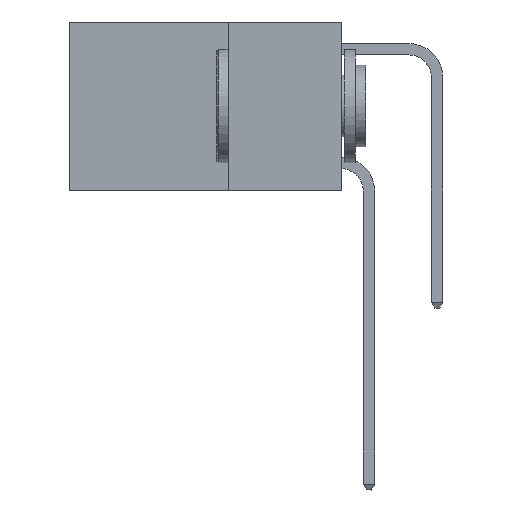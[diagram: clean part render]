
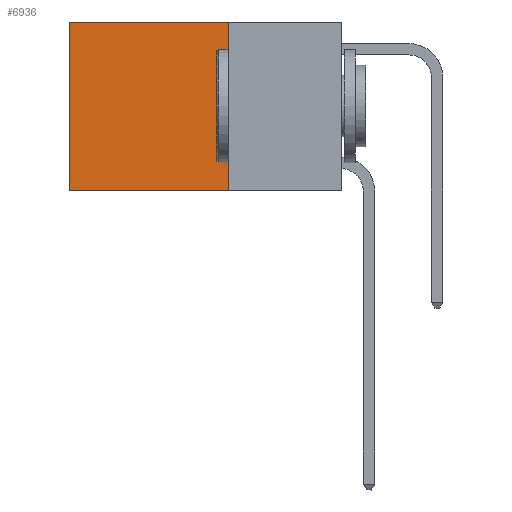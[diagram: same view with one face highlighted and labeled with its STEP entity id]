
A CAD part, left-side view. The second image highlights one B-rep face of the part: STEP entity #6936.
In plain terms, the highlighted planar face has unit normal (-1, 0, 0).
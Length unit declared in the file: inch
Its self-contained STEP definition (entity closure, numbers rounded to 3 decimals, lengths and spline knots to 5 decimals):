
#283 = CARTESIAN_POINT ( 'NONE',  ( 0.2625, 0.6, 0. ) ) ;
#607 = CARTESIAN_POINT ( 'NONE',  ( 0.2625, 0.25, 0. ) ) ;
#951 = CARTESIAN_POINT ( 'NONE',  ( 0.2625, 0.6, -0.37 ) ) ;
#1100 = VERTEX_POINT ( 'NONE', #7781 ) ;
#1145 = VERTEX_POINT ( 'NONE', #7537 ) ;
#1238 = DIRECTION ( 'NONE',  ( 1., 0., 0. ) ) ;
#1539 = VECTOR ( 'NONE', #5358, 39.37008 ) ;
#1725 = LINE ( 'NONE', #283, #9116 ) ;
#2464 = EDGE_CURVE ( 'NONE', #10876, #1145, #8487, .T. ) ;
#2500 = VERTEX_POINT ( 'NONE', #951 ) ;
#3255 = CARTESIAN_POINT ( 'NONE',  ( 0.2625, 0.25, 0. ) ) ;
#4139 = ORIENTED_EDGE ( 'NONE', *, *, #5189, .T. ) ;
#4160 = DIRECTION ( 'NONE',  ( 0., 1., 0. ) ) ;
#4683 = ORIENTED_EDGE ( 'NONE', *, *, #7695, .F. ) ;
#5189 = EDGE_CURVE ( 'NONE', #1100, #2500, #1725, .T. ) ;
#5267 = ORIENTED_EDGE ( 'NONE', *, *, #2464, .F. ) ;
#5355 = AXIS2_PLACEMENT_3D ( 'NONE', #10351, #1238, #7827 ) ;
#5358 = DIRECTION ( 'NONE',  ( 0., 1., 0. ) ) ;
#5372 = VECTOR ( 'NONE', #4160, 39.37008 ) ;
#5715 = ORIENTED_EDGE ( 'NONE', *, *, #9341, .T. ) ;
#5898 = DIRECTION ( 'NONE',  ( 0., 0., -1. ) ) ;
#6398 = VECTOR ( 'NONE', #10299, 39.37008 ) ;
#6750 = FACE_OUTER_BOUND ( 'NONE', #6798, .T. ) ;
#6798 = EDGE_LOOP ( 'NONE', ( #4139, #4683, #5267, #5715 ) ) ;
#6936 = ADVANCED_FACE ( 'NONE', ( #6750 ), #8650, .F. ) ;
#7046 = LINE ( 'NONE', #3255, #5372 ) ;
#7537 = CARTESIAN_POINT ( 'NONE',  ( 0.2625, 0.25, -0.37 ) ) ;
#7695 = EDGE_CURVE ( 'NONE', #1145, #2500, #8679, .T. ) ;
#7781 = CARTESIAN_POINT ( 'NONE',  ( 0.2625, 0.6, 0. ) ) ;
#7827 = DIRECTION ( 'NONE',  ( 0., 0., -1. ) ) ;
#8165 = CARTESIAN_POINT ( 'NONE',  ( 0.2625, 0.25, -0.37 ) ) ;
#8487 = LINE ( 'NONE', #8554, #6398 ) ;
#8554 = CARTESIAN_POINT ( 'NONE',  ( 0.2625, 0.25, 0. ) ) ;
#8650 = PLANE ( 'NONE',  #5355 ) ;
#8679 = LINE ( 'NONE', #8165, #1539 ) ;
#9116 = VECTOR ( 'NONE', #5898, 39.37008 ) ;
#9341 = EDGE_CURVE ( 'NONE', #10876, #1100, #7046, .T. ) ;
#10299 = DIRECTION ( 'NONE',  ( 0., 0., -1. ) ) ;
#10351 = CARTESIAN_POINT ( 'NONE',  ( 0.2625, 0.25, 0. ) ) ;
#10876 = VERTEX_POINT ( 'NONE', #607 ) ;
